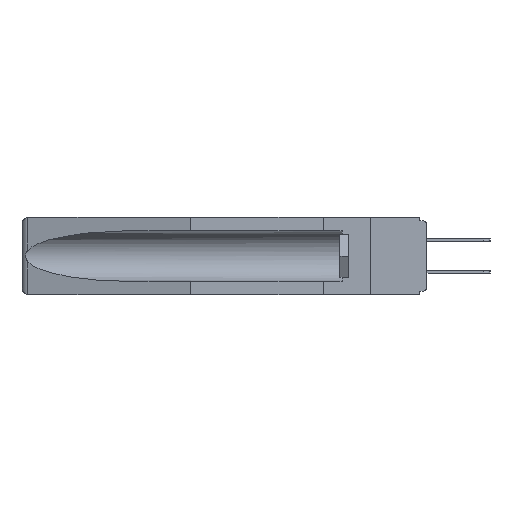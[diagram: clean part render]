
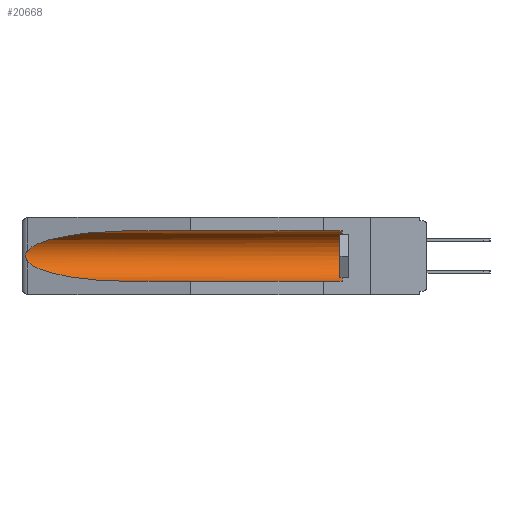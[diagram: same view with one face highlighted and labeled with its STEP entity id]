
A CAD part, left-side view. The second image highlights one B-rep face of the part: STEP entity #20668.
In plain terms, the highlighted cylindrical face has radius 2.857 mm (diameter 5.715 mm), a partial arc.
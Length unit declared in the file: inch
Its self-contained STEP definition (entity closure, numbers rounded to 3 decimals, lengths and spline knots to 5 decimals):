
#414 = ORIENTED_EDGE ( 'NONE', *, *, #7830, .F. ) ;
#1252 = CARTESIAN_POINT ( 'NONE',  ( 0.2673, 1.5327, -0.16383 ) ) ;
#1647 = CARTESIAN_POINT ( 'NONE',  ( 0.26537, 1.52718, -0.19328 ) ) ;
#2284 = CARTESIAN_POINT ( 'NONE',  ( 0.155, -0.30754, -0.059 ) ) ;
#2934 = VERTEX_POINT ( 'NONE', #1647 ) ;
#2989 = CYLINDRICAL_SURFACE ( 'NONE', #21374, 0.1125 ) ;
#3472 = CARTESIAN_POINT ( 'NONE',  ( 0.26597, 1.5296, -0.19026 ) ) ;
#3635 = DIRECTION ( 'NONE',  ( 0., 0., 1. ) ) ;
#4368 = DIRECTION ( 'NONE',  ( 0., 1., 0. ) ) ;
#5204 = EDGE_CURVE ( 'NONE', #13370, #24157, #20735, .T. ) ;
#5827 = CARTESIAN_POINT ( 'NONE',  ( 0.155, 0.126, -0.1715 ) ) ;
#6735 = ORIENTED_EDGE ( 'NONE', *, *, #5204, .T. ) ;
#7136 = CARTESIAN_POINT ( 'NONE',  ( 0.21114, 1.30732, -0.059 ) ) ;
#7275 = VERTEX_POINT ( 'NONE', #28648 ) ;
#7830 = EDGE_CURVE ( 'NONE', #7275, #21876, #13100, .T. ) ;
#8575 = VECTOR ( 'NONE', #22784, 39.37008 ) ;
#9323 = VERTEX_POINT ( 'NONE', #18021 ) ;
#9413 = CARTESIAN_POINT ( 'NONE',  ( 0.155, 1.07973, -0.059 ) ) ;
#10329 = EDGE_CURVE ( 'NONE', #9323, #2934, #24595, .T. ) ;
#10689 = CARTESIAN_POINT ( 'NONE',  ( 0.155, 1.07973, -0.284 ) ) ;
#11766 = ORIENTED_EDGE ( 'NONE', *, *, #27473, .T. ) ;
#12775 = DIRECTION ( 'NONE',  ( 0., 1., 0. ) ) ;
#12840 = EDGE_LOOP ( 'NONE', ( #17354, #18902, #11766, #414, #19358, #6735 ) ) ;
#13100 = LINE ( 'NONE', #27320, #24587 ) ;
#13370 = VERTEX_POINT ( 'NONE', #25510 ) ;
#13896 = EDGE_CURVE ( 'NONE', #24157, #9323, #19219, .T. ) ;
#14376 = CARTESIAN_POINT ( 'NONE',  ( 0.26597, 1.52961, -0.15275 ) ) ;
#14613 = CIRCLE ( 'NONE', #25280, 0.1125 ) ;
#14947 = CARTESIAN_POINT ( 'NONE',  ( 0.2675, 1.53308, -0.17534 ) ) ;
#15177 = DIRECTION ( 'NONE',  ( 0., 0., 1. ) ) ;
#16216 = CARTESIAN_POINT ( 'NONE',  ( 0.155, 1.07973, -0.059 ) ) ;
#17267 = CARTESIAN_POINT ( 'NONE',  ( 0.26655, 1.53094, -0.18657 ) ) ;
#17354 = ORIENTED_EDGE ( 'NONE', *, *, #13896, .T. ) ;
#17829 = CARTESIAN_POINT ( 'NONE',  ( 0.21114, 1.30732, -0.284 ) ) ;
#18021 = CARTESIAN_POINT ( 'NONE',  ( 0.26537, 1.52718, -0.14972 ) ) ;
#18902 = ORIENTED_EDGE ( 'NONE', *, *, #10329, .T. ) ;
#19219 =( BOUNDED_CURVE ( )  B_SPLINE_CURVE ( 3, ( #9413, #7136, #19287, #25460 ),
 .UNSPECIFIED., .F., .F. ) 
 B_SPLINE_CURVE_WITH_KNOTS ( ( 4, 4 ),
 ( 4.71239, 6.08839 ),
 .UNSPECIFIED. ) 
 CURVE ( )  GEOMETRIC_REPRESENTATION_ITEM ( )  RATIONAL_B_SPLINE_CURVE ( ( 1., 0.848, 0.848, 1. ) ) 
 REPRESENTATION_ITEM ( '' )  );
#19287 = CARTESIAN_POINT ( 'NONE',  ( 0.25451, 1.48313, -0.09465 ) ) ;
#19358 = ORIENTED_EDGE ( 'NONE', *, *, #23024, .T. ) ;
#20668 = ADVANCED_FACE ( 'NONE', ( #21229 ), #2989, .F. ) ;
#20735 = LINE ( 'NONE', #2284, #8575 ) ;
#21229 = FACE_OUTER_BOUND ( 'NONE', #12840, .T. ) ;
#21374 = AXIS2_PLACEMENT_3D ( 'NONE', #24524, #12775, #15177 ) ;
#21568 = CARTESIAN_POINT ( 'NONE',  ( 0.26537, 1.52718, -0.19328 ) ) ;
#21764 = CARTESIAN_POINT ( 'NONE',  ( 0.2675, 1.53308, -0.16763 ) ) ;
#21876 = VERTEX_POINT ( 'NONE', #22127 ) ;
#22127 = CARTESIAN_POINT ( 'NONE',  ( 0.155, 1.07973, -0.284 ) ) ;
#22784 = DIRECTION ( 'NONE',  ( 0., 1., 0. ) ) ;
#23024 = EDGE_CURVE ( 'NONE', #7275, #13370, #14613, .T. ) ;
#23312 =( BOUNDED_CURVE ( )  B_SPLINE_CURVE ( 3, ( #26882, #29206, #17829, #10689 ),
 .UNSPECIFIED., .F., .T. ) 
 B_SPLINE_CURVE_WITH_KNOTS ( ( 4, 4 ),
 ( 0.1948, 1.5708 ),
 .UNSPECIFIED. ) 
 CURVE ( )  GEOMETRIC_REPRESENTATION_ITEM ( )  RATIONAL_B_SPLINE_CURVE ( ( 1., 0.848, 0.848, 1. ) ) 
 REPRESENTATION_ITEM ( '' )  );
#23697 = CARTESIAN_POINT ( 'NONE',  ( 0.26654, 1.53092, -0.15636 ) ) ;
#24157 = VERTEX_POINT ( 'NONE', #16216 ) ;
#24524 = CARTESIAN_POINT ( 'NONE',  ( 0.155, -0.30754, -0.1715 ) ) ;
#24587 = VECTOR ( 'NONE', #4368, 39.37008 ) ;
#24595 = B_SPLINE_CURVE_WITH_KNOTS ( 'NONE', 3,
 ( #27958, #14376, #23697, #1252, #21764, #14947, #26294, #17267, #3472, #21568 ),
 .UNSPECIFIED., .F., .F.,
 ( 4, 2, 2, 2, 4 ),
 ( 0., 0.00029, 0.00058, 0.00087, 0.00117 ),
 .UNSPECIFIED. ) ;
#25280 = AXIS2_PLACEMENT_3D ( 'NONE', #5827, #26664, #3635 ) ;
#25460 = CARTESIAN_POINT ( 'NONE',  ( 0.26537, 1.52718, -0.14972 ) ) ;
#25510 = CARTESIAN_POINT ( 'NONE',  ( 0.155, 0.126, -0.059 ) ) ;
#26294 = CARTESIAN_POINT ( 'NONE',  ( 0.2673, 1.53269, -0.17917 ) ) ;
#26664 = DIRECTION ( 'NONE',  ( 0., -1., 0. ) ) ;
#26882 = CARTESIAN_POINT ( 'NONE',  ( 0.26537, 1.52718, -0.19328 ) ) ;
#27320 = CARTESIAN_POINT ( 'NONE',  ( 0.155, -0.30754, -0.284 ) ) ;
#27473 = EDGE_CURVE ( 'NONE', #2934, #21876, #23312, .T. ) ;
#27958 = CARTESIAN_POINT ( 'NONE',  ( 0.26537, 1.52718, -0.14972 ) ) ;
#28648 = CARTESIAN_POINT ( 'NONE',  ( 0.155, 0.126, -0.284 ) ) ;
#29206 = CARTESIAN_POINT ( 'NONE',  ( 0.25451, 1.48313, -0.24835 ) ) ;
